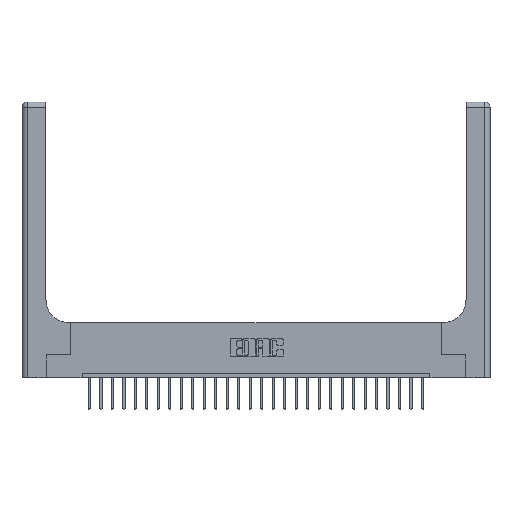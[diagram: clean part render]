
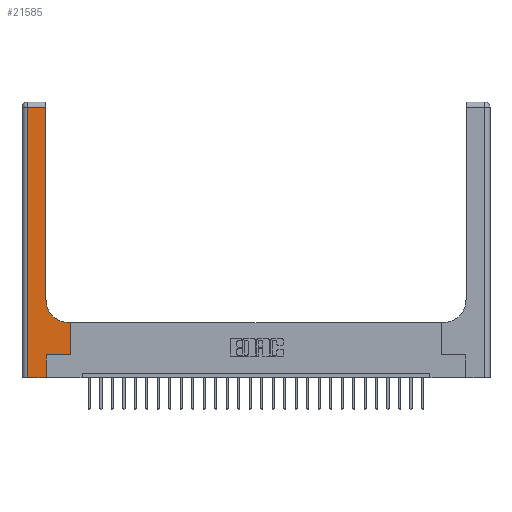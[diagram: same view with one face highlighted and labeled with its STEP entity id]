
A CAD part, top view. The second image highlights one B-rep face of the part: STEP entity #21585.
In plain terms, the highlighted planar face has unit normal (0, 0, 1).
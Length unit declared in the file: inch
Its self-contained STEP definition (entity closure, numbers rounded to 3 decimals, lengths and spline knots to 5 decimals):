
#563 = VERTEX_POINT ( 'NONE', #3246 ) ;
#853 = LINE ( 'NONE', #10789, #20810 ) ;
#1024 = VERTEX_POINT ( 'NONE', #9489 ) ;
#1080 = ORIENTED_EDGE ( 'NONE', *, *, #21273, .T. ) ;
#1314 = VECTOR ( 'NONE', #14781, 39.37008 ) ;
#1686 = VECTOR ( 'NONE', #10748, 39.37008 ) ;
#2762 = CARTESIAN_POINT ( 'NONE',  ( 0.265, 0.25, 0.37 ) ) ;
#3091 = CARTESIAN_POINT ( 'NONE',  ( 0.265, 0., 0.37 ) ) ;
#3246 = CARTESIAN_POINT ( 'NONE',  ( 0.06, 0., 0.37 ) ) ;
#3322 = EDGE_CURVE ( 'NONE', #22165, #21913, #10859, .T. ) ;
#3368 = DIRECTION ( 'NONE',  ( 1., 0., 0. ) ) ;
#4116 = CARTESIAN_POINT ( 'NONE',  ( 0.265, 0.25, 0.37 ) ) ;
#4150 = VECTOR ( 'NONE', #13047, 39.37008 ) ;
#4204 = VERTEX_POINT ( 'NONE', #23049 ) ;
#4547 = VERTEX_POINT ( 'NONE', #6799 ) ;
#4659 = DIRECTION ( 'NONE',  ( 0., -1., 0. ) ) ;
#4917 = EDGE_CURVE ( 'NONE', #563, #6374, #19038, .T. ) ;
#6374 = VERTEX_POINT ( 'NONE', #3091 ) ;
#6494 = DIRECTION ( 'NONE',  ( 1., 0., 0. ) ) ;
#6727 = EDGE_LOOP ( 'NONE', ( #14339, #17656, #12586, #22260, #17045, #20708, #14651, #14387, #1080 ) ) ;
#6743 = DIRECTION ( 'NONE',  ( -1., 0., 0. ) ) ;
#6799 = CARTESIAN_POINT ( 'NONE',  ( 0.06, 2.94, 0.37 ) ) ;
#7351 = AXIS2_PLACEMENT_3D ( 'NONE', #10957, #9367, #3368 ) ;
#7784 = VECTOR ( 'NONE', #18647, 39.37008 ) ;
#9322 = EDGE_CURVE ( 'NONE', #4204, #23636, #20353, .T. ) ;
#9367 = DIRECTION ( 'NONE',  ( 0., 0., -1. ) ) ;
#9489 = CARTESIAN_POINT ( 'NONE',  ( 0.528, 0.25, 0.37 ) ) ;
#9956 = DIRECTION ( 'NONE',  ( -1., 0., 0. ) ) ;
#10310 = LINE ( 'NONE', #10444, #19109 ) ;
#10419 = CARTESIAN_POINT ( 'NONE',  ( 0., 2.94, 0.37 ) ) ;
#10444 = CARTESIAN_POINT ( 'NONE',  ( 0.265, 0., 0.37 ) ) ;
#10748 = DIRECTION ( 'NONE',  ( 1., 0., 0. ) ) ;
#10789 = CARTESIAN_POINT ( 'NONE',  ( 0.06, 3., 0.37 ) ) ;
#10859 = LINE ( 'NONE', #10984, #1314 ) ;
#10957 = CARTESIAN_POINT ( 'NONE',  ( 0.51, 0.85, 0.37 ) ) ;
#10984 = CARTESIAN_POINT ( 'NONE',  ( 0.26, 3., 0.37 ) ) ;
#11581 = CARTESIAN_POINT ( 'NONE',  ( 0.528, 0.25, 0.37 ) ) ;
#11896 = EDGE_CURVE ( 'NONE', #1024, #4204, #22967, .T. ) ;
#12200 = CARTESIAN_POINT ( 'NONE',  ( 0., 3., 0.37 ) ) ;
#12586 = ORIENTED_EDGE ( 'NONE', *, *, #25110, .T. ) ;
#13047 = DIRECTION ( 'NONE',  ( 0., 1., 0. ) ) ;
#13977 = DIRECTION ( 'NONE',  ( 0., 1., 0. ) ) ;
#14010 = VECTOR ( 'NONE', #6743, 39.37008 ) ;
#14282 = DIRECTION ( 'NONE',  ( 0., 0., -1. ) ) ;
#14339 = ORIENTED_EDGE ( 'NONE', *, *, #3322, .T. ) ;
#14387 = ORIENTED_EDGE ( 'NONE', *, *, #9322, .T. ) ;
#14398 = FACE_OUTER_BOUND ( 'NONE', #6727, .T. ) ;
#14483 = CARTESIAN_POINT ( 'NONE',  ( 0.26, 0.6, 0.37 ) ) ;
#14651 = ORIENTED_EDGE ( 'NONE', *, *, #11896, .T. ) ;
#14781 = DIRECTION ( 'NONE',  ( 0., 1., 0. ) ) ;
#15665 = VERTEX_POINT ( 'NONE', #4116 ) ;
#16102 = PLANE ( 'NONE',  #21149 ) ;
#16837 = CARTESIAN_POINT ( 'NONE',  ( 0., 0., 0.37 ) ) ;
#17045 = ORIENTED_EDGE ( 'NONE', *, *, #24722, .T. ) ;
#17384 = CARTESIAN_POINT ( 'NONE',  ( 0.26, 2.94, 0.37 ) ) ;
#17531 = EDGE_CURVE ( 'NONE', #15665, #1024, #20679, .T. ) ;
#17656 = ORIENTED_EDGE ( 'NONE', *, *, #20012, .T. ) ;
#18647 = DIRECTION ( 'NONE',  ( -1., 0., 0. ) ) ;
#19038 = LINE ( 'NONE', #16837, #22102 ) ;
#19109 = VECTOR ( 'NONE', #13977, 39.37008 ) ;
#19825 = CARTESIAN_POINT ( 'NONE',  ( 0.51, 0.6, 0.37 ) ) ;
#20012 = EDGE_CURVE ( 'NONE', #21913, #4547, #22301, .T. ) ;
#20353 = LINE ( 'NONE', #14483, #7784 ) ;
#20679 = LINE ( 'NONE', #2762, #1686 ) ;
#20708 = ORIENTED_EDGE ( 'NONE', *, *, #17531, .T. ) ;
#20810 = VECTOR ( 'NONE', #4659, 39.37008 ) ;
#21149 = AXIS2_PLACEMENT_3D ( 'NONE', #12200, #14282, #9956 ) ;
#21273 = EDGE_CURVE ( 'NONE', #23636, #22165, #22412, .T. ) ;
#21585 = ADVANCED_FACE ( 'NONE', ( #14398 ), #16102, .F. ) ;
#21913 = VERTEX_POINT ( 'NONE', #17384 ) ;
#22102 = VECTOR ( 'NONE', #6494, 39.37008 ) ;
#22165 = VERTEX_POINT ( 'NONE', #22330 ) ;
#22260 = ORIENTED_EDGE ( 'NONE', *, *, #4917, .T. ) ;
#22301 = LINE ( 'NONE', #10419, #14010 ) ;
#22330 = CARTESIAN_POINT ( 'NONE',  ( 0.26, 0.85, 0.37 ) ) ;
#22412 = CIRCLE ( 'NONE', #7351, 0.25 ) ;
#22967 = LINE ( 'NONE', #11581, #4150 ) ;
#23049 = CARTESIAN_POINT ( 'NONE',  ( 0.528, 0.6, 0.37 ) ) ;
#23636 = VERTEX_POINT ( 'NONE', #19825 ) ;
#24722 = EDGE_CURVE ( 'NONE', #6374, #15665, #10310, .T. ) ;
#25110 = EDGE_CURVE ( 'NONE', #4547, #563, #853, .T. ) ;
